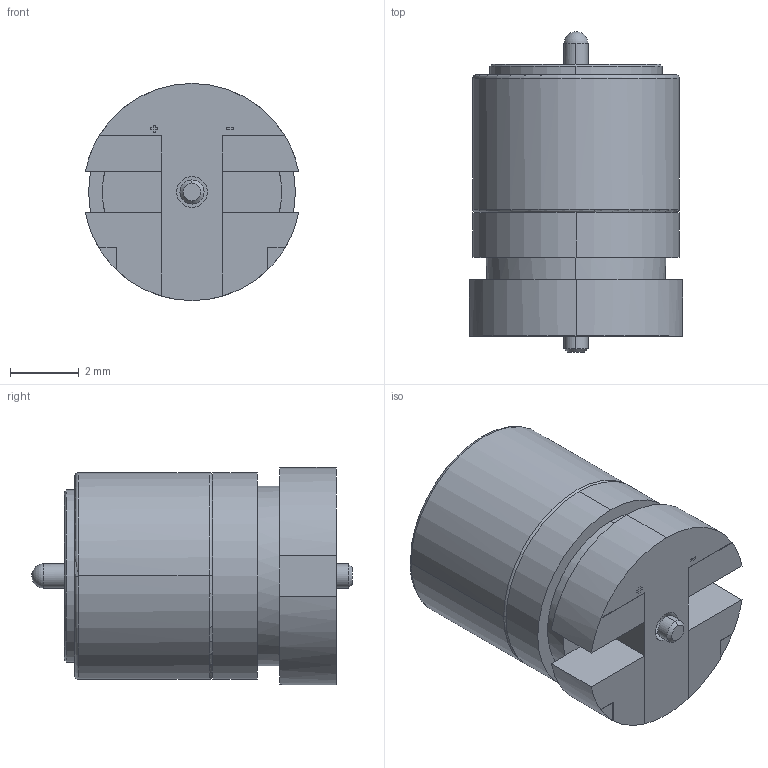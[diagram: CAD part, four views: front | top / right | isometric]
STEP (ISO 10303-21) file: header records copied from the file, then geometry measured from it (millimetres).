
FILE_DESCRIPTION (( 'STEP AP214' ), '1' );
FILE_NAME ('685B0212P011B0E.STEP', '2023-08-15T15:44:38', ( '' ), ( '' ), 'SwSTEP 2.0', 'SolidWorks 2023', '' );
FILE_SCHEMA (( 'AUTOMOTIVE_DESIGN' ));
Length unit declared in the file: millimetre
Products named in the file (1): 685B0212P011B0E
Bounding box: 6.18 x 9.3 x 6.3 mm (x, y, z)
Volume: 210.5 mm3; surface area: 254.5 mm2
Topology: 2 solids, 4 shells, 95 faces, 238 edges, 156 vertices
Faces by surface type: plane 55, cylinder 25, torus 10, cone 4, sphere 1
Entity records: 2887 total; most frequent: DIRECTION 525, CARTESIAN_POINT 487, ORIENTED_EDGE 472, EDGE_CURVE 236, AXIS2_PLACEMENT_3D 193, VERTEX_POINT 155, LINE 139, VECTOR 139
